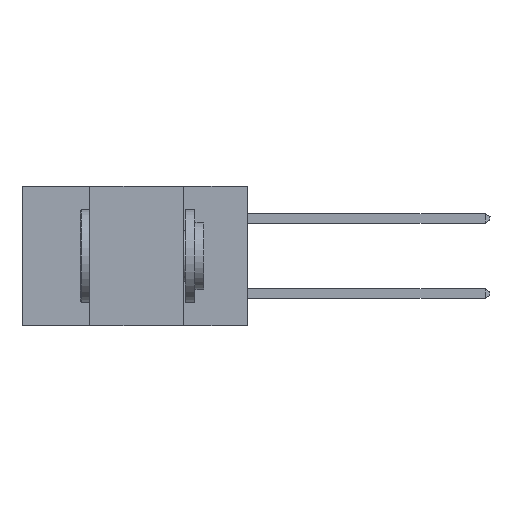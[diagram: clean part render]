
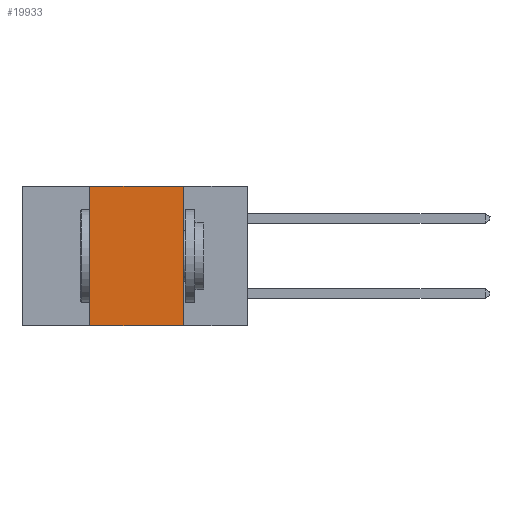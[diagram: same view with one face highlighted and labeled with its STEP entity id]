
A CAD part, left-side view. The second image highlights one B-rep face of the part: STEP entity #19933.
In plain terms, the highlighted planar face has unit normal (-1, 0, 0).
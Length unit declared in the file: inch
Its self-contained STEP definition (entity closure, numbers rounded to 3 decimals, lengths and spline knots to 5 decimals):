
#975 = PLANE ( 'NONE',  #7156 ) ;
#1580 = VERTEX_POINT ( 'NONE', #9726 ) ;
#2703 = VECTOR ( 'NONE', #19747, 39.37008 ) ;
#4490 = CARTESIAN_POINT ( 'NONE',  ( 0., 0.42, -0.37 ) ) ;
#4935 = EDGE_CURVE ( 'NONE', #1580, #5786, #7121, .T. ) ;
#5786 = VERTEX_POINT ( 'NONE', #10621 ) ;
#5969 = VERTEX_POINT ( 'NONE', #19487 ) ;
#6001 = CARTESIAN_POINT ( 'NONE',  ( 0., 0.6, 0. ) ) ;
#7121 = LINE ( 'NONE', #11917, #2703 ) ;
#7156 = AXIS2_PLACEMENT_3D ( 'NONE', #6001, #17363, #7668 ) ;
#7668 = DIRECTION ( 'NONE',  ( 0., 0., -1. ) ) ;
#7683 = FACE_OUTER_BOUND ( 'NONE', #16139, .T. ) ;
#8889 = VECTOR ( 'NONE', #10663, 39.37008 ) ;
#9149 = DIRECTION ( 'NONE',  ( 0., -1., 0. ) ) ;
#9726 = CARTESIAN_POINT ( 'NONE',  ( 0., 0.17, 0. ) ) ;
#10621 = CARTESIAN_POINT ( 'NONE',  ( 0., 0.17, -0.37 ) ) ;
#10648 = LINE ( 'NONE', #20324, #8889 ) ;
#10663 = DIRECTION ( 'NONE',  ( 0., 0., 1. ) ) ;
#11559 = EDGE_CURVE ( 'NONE', #16542, #5786, #17622, .T. ) ;
#11917 = CARTESIAN_POINT ( 'NONE',  ( 0., 0.17, 0. ) ) ;
#13080 = CARTESIAN_POINT ( 'NONE',  ( 0., 0.6, 0. ) ) ;
#13688 = EDGE_CURVE ( 'NONE', #5969, #1580, #20357, .T. ) ;
#13770 = VECTOR ( 'NONE', #9149, 39.37008 ) ;
#14737 = DIRECTION ( 'NONE',  ( 0., -1., 0. ) ) ;
#14847 = ORIENTED_EDGE ( 'NONE', *, *, #13688, .F. ) ;
#15229 = ORIENTED_EDGE ( 'NONE', *, *, #11559, .T. ) ;
#15280 = ORIENTED_EDGE ( 'NONE', *, *, #16340, .F. ) ;
#15428 = ORIENTED_EDGE ( 'NONE', *, *, #4935, .F. ) ;
#16139 = EDGE_LOOP ( 'NONE', ( #15428, #14847, #15280, #15229 ) ) ;
#16340 = EDGE_CURVE ( 'NONE', #16542, #5969, #10648, .T. ) ;
#16542 = VERTEX_POINT ( 'NONE', #4490 ) ;
#17363 = DIRECTION ( 'NONE',  ( 1., 0., 0. ) ) ;
#17622 = LINE ( 'NONE', #18826, #13770 ) ;
#18826 = CARTESIAN_POINT ( 'NONE',  ( 0., 0.6, -0.37 ) ) ;
#19487 = CARTESIAN_POINT ( 'NONE',  ( 0., 0.42, 0. ) ) ;
#19747 = DIRECTION ( 'NONE',  ( 0., 0., -1. ) ) ;
#19867 = VECTOR ( 'NONE', #14737, 39.37008 ) ;
#19933 = ADVANCED_FACE ( 'NONE', ( #7683 ), #975, .F. ) ;
#20324 = CARTESIAN_POINT ( 'NONE',  ( 0., 0.42, 0. ) ) ;
#20357 = LINE ( 'NONE', #13080, #19867 ) ;
